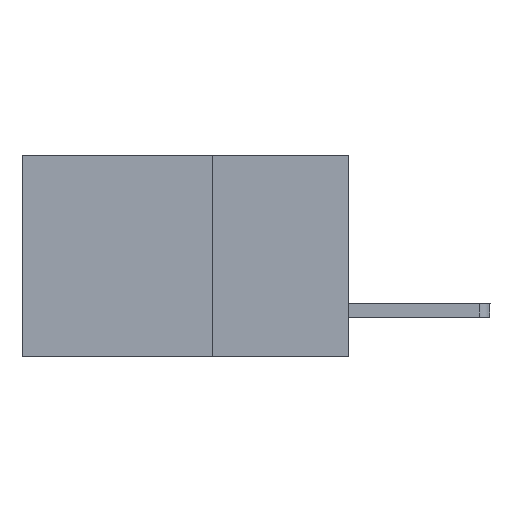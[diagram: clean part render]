
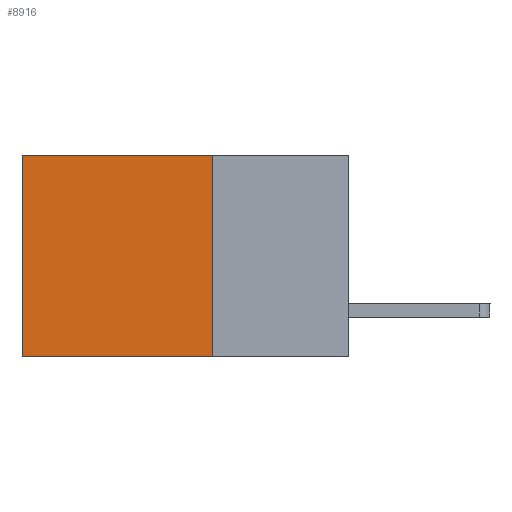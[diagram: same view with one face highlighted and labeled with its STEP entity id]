
A CAD part, left-side view. The second image highlights one B-rep face of the part: STEP entity #8916.
In plain terms, the highlighted planar face has unit normal (-1, 0, 0).
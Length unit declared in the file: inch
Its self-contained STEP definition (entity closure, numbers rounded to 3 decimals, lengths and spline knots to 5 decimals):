
#26 = DIRECTION ( 'NONE',  ( 0., 0., -1. ) ) ;
#192 = VERTEX_POINT ( 'NONE', #1148 ) ;
#218 = CARTESIAN_POINT ( 'NONE',  ( 0.298, 0.25, 0. ) ) ;
#335 = VECTOR ( 'NONE', #2262, 39.37008 ) ;
#458 = LINE ( 'NONE', #10234, #10257 ) ;
#459 = VERTEX_POINT ( 'NONE', #8588 ) ;
#895 = PLANE ( 'NONE',  #9492 ) ;
#1005 = DIRECTION ( 'NONE',  ( 0., 1., 0. ) ) ;
#1148 = CARTESIAN_POINT ( 'NONE',  ( 0.298, 0.25, -0.37 ) ) ;
#1566 = DIRECTION ( 'NONE',  ( 1., 0., 0. ) ) ;
#1675 = ORIENTED_EDGE ( 'NONE', *, *, #1943, .F. ) ;
#1707 = LINE ( 'NONE', #218, #6654 ) ;
#1793 = FACE_OUTER_BOUND ( 'NONE', #2355, .T. ) ;
#1895 = EDGE_CURVE ( 'NONE', #459, #5725, #458, .T. ) ;
#1943 = EDGE_CURVE ( 'NONE', #9563, #192, #3955, .T. ) ;
#2262 = DIRECTION ( 'NONE',  ( 0., 0., -1. ) ) ;
#2355 = EDGE_LOOP ( 'NONE', ( #4472, #4289, #1675, #7995 ) ) ;
#2617 = DIRECTION ( 'NONE',  ( 0., 1., 0. ) ) ;
#3885 = VECTOR ( 'NONE', #2617, 39.37008 ) ;
#3955 = LINE ( 'NONE', #7885, #335 ) ;
#4289 = ORIENTED_EDGE ( 'NONE', *, *, #4294, .F. ) ;
#4294 = EDGE_CURVE ( 'NONE', #192, #5725, #7337, .T. ) ;
#4472 = ORIENTED_EDGE ( 'NONE', *, *, #1895, .T. ) ;
#4872 = CARTESIAN_POINT ( 'NONE',  ( 0.298, 0.6, -0.37 ) ) ;
#5510 = DIRECTION ( 'NONE',  ( 0., 0., -1. ) ) ;
#5725 = VERTEX_POINT ( 'NONE', #4872 ) ;
#6654 = VECTOR ( 'NONE', #1005, 39.37008 ) ;
#6929 = CARTESIAN_POINT ( 'NONE',  ( 0.298, 0.25, 0. ) ) ;
#7337 = LINE ( 'NONE', #9044, #3885 ) ;
#7885 = CARTESIAN_POINT ( 'NONE',  ( 0.298, 0.25, 0. ) ) ;
#7995 = ORIENTED_EDGE ( 'NONE', *, *, #9663, .T. ) ;
#8588 = CARTESIAN_POINT ( 'NONE',  ( 0.298, 0.6, 0. ) ) ;
#8916 = ADVANCED_FACE ( 'NONE', ( #1793 ), #895, .F. ) ;
#9044 = CARTESIAN_POINT ( 'NONE',  ( 0.298, 0.25, -0.37 ) ) ;
#9492 = AXIS2_PLACEMENT_3D ( 'NONE', #9569, #1566, #26 ) ;
#9563 = VERTEX_POINT ( 'NONE', #6929 ) ;
#9569 = CARTESIAN_POINT ( 'NONE',  ( 0.298, 0.25, 0. ) ) ;
#9663 = EDGE_CURVE ( 'NONE', #9563, #459, #1707, .T. ) ;
#10234 = CARTESIAN_POINT ( 'NONE',  ( 0.298, 0.6, 0. ) ) ;
#10257 = VECTOR ( 'NONE', #5510, 39.37008 ) ;
